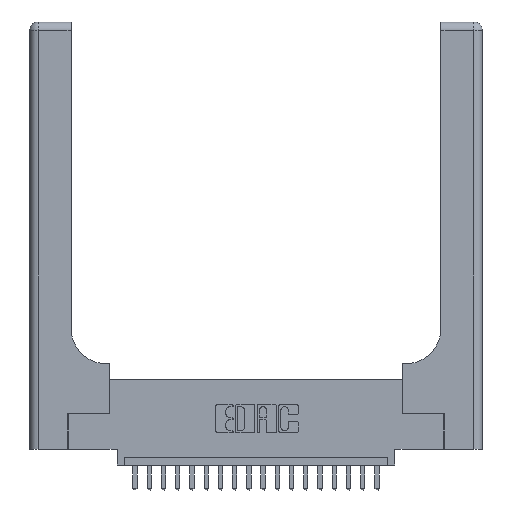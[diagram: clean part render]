
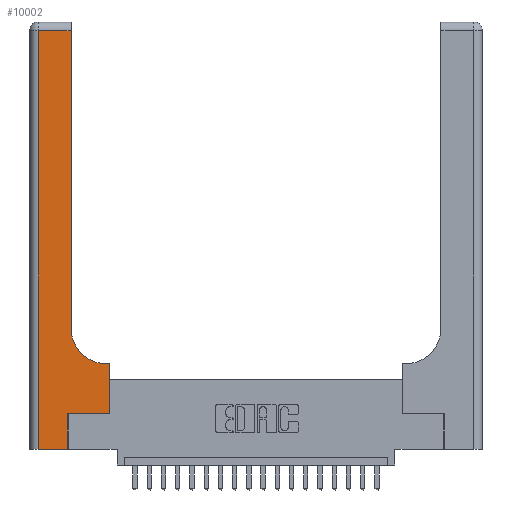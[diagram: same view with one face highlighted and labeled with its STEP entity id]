
A CAD part, top view. The second image highlights one B-rep face of the part: STEP entity #10002.
In plain terms, the highlighted planar face has unit normal (0, 0, 1).
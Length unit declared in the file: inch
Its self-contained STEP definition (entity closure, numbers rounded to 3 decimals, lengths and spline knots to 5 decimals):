
#412 = DIRECTION ( 'NONE',  ( 0., 1., 0. ) ) ;
#633 = VECTOR ( 'NONE', #8733, 39.37008 ) ;
#834 = CARTESIAN_POINT ( 'NONE',  ( 0.2915, 0.6, 0.37 ) ) ;
#1003 = CARTESIAN_POINT ( 'NONE',  ( 0., 0., 0.37 ) ) ;
#1330 = CARTESIAN_POINT ( 'NONE',  ( 0.269, 0., 0.37 ) ) ;
#1701 = CARTESIAN_POINT ( 'NONE',  ( 0.269, 0.25, 0.37 ) ) ;
#1789 = CARTESIAN_POINT ( 'NONE',  ( 0.5585, 0.6, 0.37 ) ) ;
#1996 = LINE ( 'NONE', #1003, #16181 ) ;
#2050 = VECTOR ( 'NONE', #412, 39.37008 ) ;
#2296 = FACE_OUTER_BOUND ( 'NONE', #4225, .T. ) ;
#2410 = EDGE_CURVE ( 'NONE', #9364, #7230, #19414, .T. ) ;
#2630 = DIRECTION ( 'NONE',  ( -1., 0., 0. ) ) ;
#3581 = CARTESIAN_POINT ( 'NONE',  ( 0.2915, 3., 0.37 ) ) ;
#3666 = ORIENTED_EDGE ( 'NONE', *, *, #16803, .T. ) ;
#3984 = EDGE_CURVE ( 'NONE', #4992, #17961, #10509, .T. ) ;
#4203 = LINE ( 'NONE', #834, #21640 ) ;
#4225 = EDGE_LOOP ( 'NONE', ( #14492, #14745, #3666, #18933, #6424, #14022, #8204, #6127, #8772 ) ) ;
#4992 = VERTEX_POINT ( 'NONE', #13698 ) ;
#5275 = CARTESIAN_POINT ( 'NONE',  ( 0.06, 3., 0.37 ) ) ;
#5443 = CARTESIAN_POINT ( 'NONE',  ( 0.269, 0., 0.37 ) ) ;
#5775 = CARTESIAN_POINT ( 'NONE',  ( 0.269, 0.25, 0.37 ) ) ;
#5855 = DIRECTION ( 'NONE',  ( 1., 0., 0. ) ) ;
#5981 = CARTESIAN_POINT ( 'NONE',  ( 0.5415, 0.85, 0.37 ) ) ;
#6127 = ORIENTED_EDGE ( 'NONE', *, *, #15319, .T. ) ;
#6424 = ORIENTED_EDGE ( 'NONE', *, *, #21222, .T. ) ;
#6693 = EDGE_CURVE ( 'NONE', #7450, #4992, #12890, .T. ) ;
#7230 = VERTEX_POINT ( 'NONE', #21717 ) ;
#7450 = VERTEX_POINT ( 'NONE', #20460 ) ;
#7646 = LINE ( 'NONE', #1330, #21598 ) ;
#8204 = ORIENTED_EDGE ( 'NONE', *, *, #9423, .T. ) ;
#8337 = VERTEX_POINT ( 'NONE', #11173 ) ;
#8733 = DIRECTION ( 'NONE',  ( 0., -1., 0. ) ) ;
#8772 = ORIENTED_EDGE ( 'NONE', *, *, #6693, .T. ) ;
#9364 = VERTEX_POINT ( 'NONE', #1701 ) ;
#9423 = EDGE_CURVE ( 'NONE', #7230, #11831, #16502, .T. ) ;
#9486 = LINE ( 'NONE', #5275, #633 ) ;
#9624 = AXIS2_PLACEMENT_3D ( 'NONE', #17013, #20467, #18741 ) ;
#10002 = ADVANCED_FACE ( 'NONE', ( #2296 ), #15225, .F. ) ;
#10466 = DIRECTION ( 'NONE',  ( -1., 0., 0. ) ) ;
#10509 = LINE ( 'NONE', #3581, #19072 ) ;
#11173 = CARTESIAN_POINT ( 'NONE',  ( 0.06, 2.94, 0.37 ) ) ;
#11258 = DIRECTION ( 'NONE',  ( 1., 0., 0. ) ) ;
#11831 = VERTEX_POINT ( 'NONE', #1789 ) ;
#12040 = DIRECTION ( 'NONE',  ( 0., 1., 0. ) ) ;
#12407 = CARTESIAN_POINT ( 'NONE',  ( 0.2915, 2.94, 0.37 ) ) ;
#12703 = VECTOR ( 'NONE', #5855, 39.37008 ) ;
#12775 = DIRECTION ( 'NONE',  ( 1., 0., 0. ) ) ;
#12890 = CIRCLE ( 'NONE', #22067, 0.25 ) ;
#13303 = DIRECTION ( 'NONE',  ( 0., 1., 0. ) ) ;
#13698 = CARTESIAN_POINT ( 'NONE',  ( 0.2915, 0.85, 0.37 ) ) ;
#14022 = ORIENTED_EDGE ( 'NONE', *, *, #2410, .T. ) ;
#14492 = ORIENTED_EDGE ( 'NONE', *, *, #3984, .T. ) ;
#14524 = DIRECTION ( 'NONE',  ( 0., 0., -1. ) ) ;
#14745 = ORIENTED_EDGE ( 'NONE', *, *, #18431, .T. ) ;
#15225 = PLANE ( 'NONE',  #9624 ) ;
#15319 = EDGE_CURVE ( 'NONE', #11831, #7450, #4203, .T. ) ;
#15616 = VERTEX_POINT ( 'NONE', #5443 ) ;
#16181 = VECTOR ( 'NONE', #11258, 39.37008 ) ;
#16502 = LINE ( 'NONE', #17617, #2050 ) ;
#16803 = EDGE_CURVE ( 'NONE', #8337, #17053, #9486, .T. ) ;
#16902 = VECTOR ( 'NONE', #10466, 39.37008 ) ;
#17013 = CARTESIAN_POINT ( 'NONE',  ( 0., 3., 0.37 ) ) ;
#17053 = VERTEX_POINT ( 'NONE', #21698 ) ;
#17617 = CARTESIAN_POINT ( 'NONE',  ( 0.5585, 0.25, 0.37 ) ) ;
#17961 = VERTEX_POINT ( 'NONE', #12407 ) ;
#18431 = EDGE_CURVE ( 'NONE', #17961, #8337, #21487, .T. ) ;
#18741 = DIRECTION ( 'NONE',  ( -1., 0., 0. ) ) ;
#18933 = ORIENTED_EDGE ( 'NONE', *, *, #21699, .T. ) ;
#19072 = VECTOR ( 'NONE', #12040, 39.37008 ) ;
#19414 = LINE ( 'NONE', #5775, #12703 ) ;
#20460 = CARTESIAN_POINT ( 'NONE',  ( 0.5415, 0.6, 0.37 ) ) ;
#20467 = DIRECTION ( 'NONE',  ( 0., 0., -1. ) ) ;
#20725 = CARTESIAN_POINT ( 'NONE',  ( 0., 2.94, 0.37 ) ) ;
#21222 = EDGE_CURVE ( 'NONE', #15616, #9364, #7646, .T. ) ;
#21487 = LINE ( 'NONE', #20725, #16902 ) ;
#21598 = VECTOR ( 'NONE', #13303, 39.37008 ) ;
#21640 = VECTOR ( 'NONE', #2630, 39.37008 ) ;
#21698 = CARTESIAN_POINT ( 'NONE',  ( 0.06, 0., 0.37 ) ) ;
#21699 = EDGE_CURVE ( 'NONE', #17053, #15616, #1996, .T. ) ;
#21717 = CARTESIAN_POINT ( 'NONE',  ( 0.5585, 0.25, 0.37 ) ) ;
#22067 = AXIS2_PLACEMENT_3D ( 'NONE', #5981, #14524, #12775 ) ;
